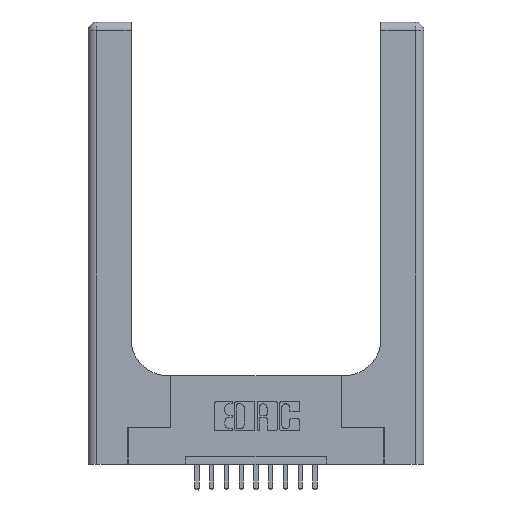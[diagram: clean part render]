
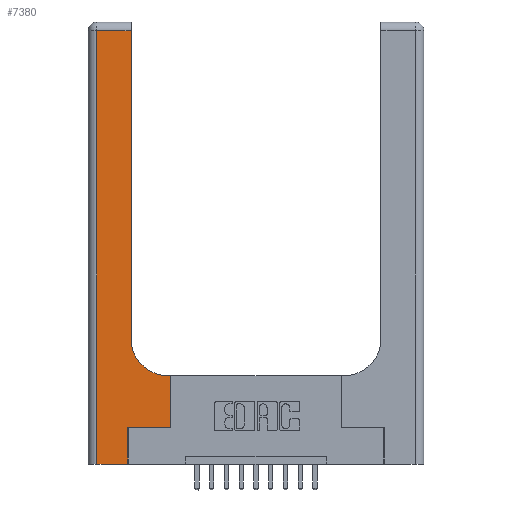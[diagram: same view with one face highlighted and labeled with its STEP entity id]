
A CAD part, top view. The second image highlights one B-rep face of the part: STEP entity #7380.
In plain terms, the highlighted planar face has unit normal (0, 0, 1).
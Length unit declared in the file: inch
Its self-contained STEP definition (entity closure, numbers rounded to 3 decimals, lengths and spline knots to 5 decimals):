
#388 = ORIENTED_EDGE ( 'NONE', *, *, #13421, .T. ) ;
#1362 = ORIENTED_EDGE ( 'NONE', *, *, #14070, .T. ) ;
#1622 = CARTESIAN_POINT ( 'NONE',  ( 0.06, 0., 0.37 ) ) ;
#1636 = DIRECTION ( 'NONE',  ( 1., 0., 0. ) ) ;
#1670 = CARTESIAN_POINT ( 'NONE',  ( 0.5585, 0.25, 0.37 ) ) ;
#1808 = CARTESIAN_POINT ( 'NONE',  ( 0., 3., 0.37 ) ) ;
#1963 = ORIENTED_EDGE ( 'NONE', *, *, #6804, .T. ) ;
#1974 = VERTEX_POINT ( 'NONE', #13988 ) ;
#1976 = DIRECTION ( 'NONE',  ( -1., 0., 0. ) ) ;
#2103 = VECTOR ( 'NONE', #8853, 39.37008 ) ;
#2857 = ORIENTED_EDGE ( 'NONE', *, *, #8823, .T. ) ;
#2942 = DIRECTION ( 'NONE',  ( 1., 0., 0. ) ) ;
#3116 = CARTESIAN_POINT ( 'NONE',  ( 0.2915, 2.94, 0.37 ) ) ;
#3151 = ORIENTED_EDGE ( 'NONE', *, *, #5465, .T. ) ;
#3268 = DIRECTION ( 'NONE',  ( 0., -1., 0. ) ) ;
#3417 = VERTEX_POINT ( 'NONE', #1670 ) ;
#3940 = LINE ( 'NONE', #9894, #4334 ) ;
#4100 = CARTESIAN_POINT ( 'NONE',  ( 0.269, 0., 0.37 ) ) ;
#4334 = VECTOR ( 'NONE', #7590, 39.37008 ) ;
#4676 = LINE ( 'NONE', #9377, #11433 ) ;
#5100 = EDGE_LOOP ( 'NONE', ( #8093, #10951, #1362, #9246, #2857, #388, #1963, #5557, #3151 ) ) ;
#5229 = CARTESIAN_POINT ( 'NONE',  ( 0.269, 0., 0.37 ) ) ;
#5465 = EDGE_CURVE ( 'NONE', #11272, #11916, #13461, .T. ) ;
#5555 = CARTESIAN_POINT ( 'NONE',  ( 0.269, 0.25, 0.37 ) ) ;
#5557 = ORIENTED_EDGE ( 'NONE', *, *, #15078, .T. ) ;
#6277 = VECTOR ( 'NONE', #9161, 39.37008 ) ;
#6804 = EDGE_CURVE ( 'NONE', #3417, #1974, #3940, .T. ) ;
#7205 = LINE ( 'NONE', #8707, #15718 ) ;
#7297 = VERTEX_POINT ( 'NONE', #1622 ) ;
#7380 = ADVANCED_FACE ( 'NONE', ( #14087 ), #15802, .F. ) ;
#7590 = DIRECTION ( 'NONE',  ( 0., 1., 0. ) ) ;
#7790 = EDGE_CURVE ( 'NONE', #7297, #14017, #12083, .T. ) ;
#7797 = CARTESIAN_POINT ( 'NONE',  ( 0.5415, 0.85, 0.37 ) ) ;
#8014 = VECTOR ( 'NONE', #14425, 39.37008 ) ;
#8018 = DIRECTION ( 'NONE',  ( 0., 0., -1. ) ) ;
#8093 = ORIENTED_EDGE ( 'NONE', *, *, #9369, .T. ) ;
#8538 = CARTESIAN_POINT ( 'NONE',  ( 0.2915, 0.85, 0.37 ) ) ;
#8707 = CARTESIAN_POINT ( 'NONE',  ( 0., 2.94, 0.37 ) ) ;
#8823 = EDGE_CURVE ( 'NONE', #14017, #12555, #13051, .T. ) ;
#8830 = DIRECTION ( 'NONE',  ( 0., 1., 0. ) ) ;
#8853 = DIRECTION ( 'NONE',  ( 0., 1., 0. ) ) ;
#8927 = LINE ( 'NONE', #5555, #13125 ) ;
#9161 = DIRECTION ( 'NONE',  ( 1., 0., 0. ) ) ;
#9194 = AXIS2_PLACEMENT_3D ( 'NONE', #7797, #8018, #1636 ) ;
#9246 = ORIENTED_EDGE ( 'NONE', *, *, #7790, .T. ) ;
#9369 = EDGE_CURVE ( 'NONE', #11916, #15059, #12832, .T. ) ;
#9377 = CARTESIAN_POINT ( 'NONE',  ( 0.06, 3., 0.37 ) ) ;
#9425 = LINE ( 'NONE', #14483, #8014 ) ;
#9805 = CARTESIAN_POINT ( 'NONE',  ( 0.269, 0.25, 0.37 ) ) ;
#9894 = CARTESIAN_POINT ( 'NONE',  ( 0.5585, 0.25, 0.37 ) ) ;
#10951 = ORIENTED_EDGE ( 'NONE', *, *, #13651, .T. ) ;
#11272 = VERTEX_POINT ( 'NONE', #13552 ) ;
#11433 = VECTOR ( 'NONE', #3268, 39.37008 ) ;
#11493 = CARTESIAN_POINT ( 'NONE',  ( 0., 0., 0.37 ) ) ;
#11604 = VECTOR ( 'NONE', #8830, 39.37008 ) ;
#11916 = VERTEX_POINT ( 'NONE', #8538 ) ;
#11981 = DIRECTION ( 'NONE',  ( 0., 0., -1. ) ) ;
#12083 = LINE ( 'NONE', #11493, #6277 ) ;
#12103 = AXIS2_PLACEMENT_3D ( 'NONE', #1808, #11981, #1976 ) ;
#12555 = VERTEX_POINT ( 'NONE', #9805 ) ;
#12832 = LINE ( 'NONE', #16505, #11604 ) ;
#12925 = CARTESIAN_POINT ( 'NONE',  ( 0.06, 2.94, 0.37 ) ) ;
#13051 = LINE ( 'NONE', #5229, #2103 ) ;
#13125 = VECTOR ( 'NONE', #2942, 39.37008 ) ;
#13319 = VERTEX_POINT ( 'NONE', #12925 ) ;
#13421 = EDGE_CURVE ( 'NONE', #12555, #3417, #8927, .T. ) ;
#13461 = CIRCLE ( 'NONE', #9194, 0.25 ) ;
#13552 = CARTESIAN_POINT ( 'NONE',  ( 0.5415, 0.6, 0.37 ) ) ;
#13651 = EDGE_CURVE ( 'NONE', #15059, #13319, #7205, .T. ) ;
#13988 = CARTESIAN_POINT ( 'NONE',  ( 0.5585, 0.6, 0.37 ) ) ;
#14017 = VERTEX_POINT ( 'NONE', #4100 ) ;
#14070 = EDGE_CURVE ( 'NONE', #13319, #7297, #4676, .T. ) ;
#14087 = FACE_OUTER_BOUND ( 'NONE', #5100, .T. ) ;
#14425 = DIRECTION ( 'NONE',  ( -1., 0., 0. ) ) ;
#14483 = CARTESIAN_POINT ( 'NONE',  ( 0.2915, 0.6, 0.37 ) ) ;
#15059 = VERTEX_POINT ( 'NONE', #3116 ) ;
#15078 = EDGE_CURVE ( 'NONE', #1974, #11272, #9425, .T. ) ;
#15109 = DIRECTION ( 'NONE',  ( -1., 0., 0. ) ) ;
#15718 = VECTOR ( 'NONE', #15109, 39.37008 ) ;
#15802 = PLANE ( 'NONE',  #12103 ) ;
#16505 = CARTESIAN_POINT ( 'NONE',  ( 0.2915, 3., 0.37 ) ) ;
